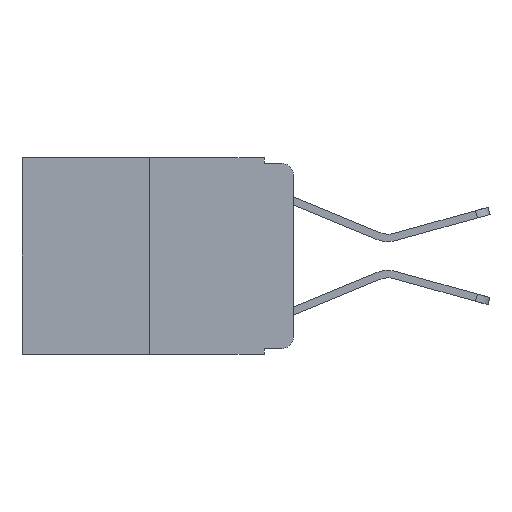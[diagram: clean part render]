
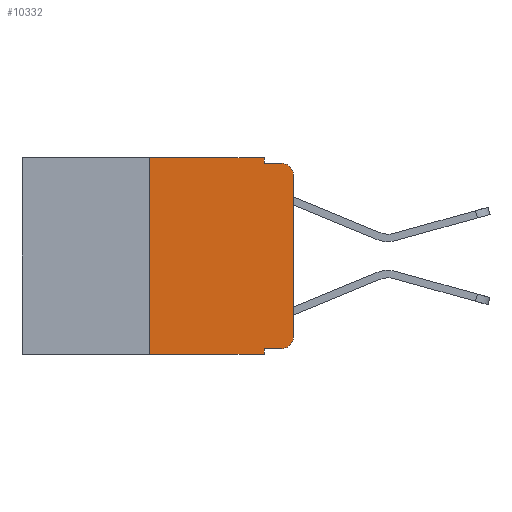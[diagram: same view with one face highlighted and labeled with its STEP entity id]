
A CAD part, left-side view. The second image highlights one B-rep face of the part: STEP entity #10332.
In plain terms, the highlighted planar face has unit normal (-1, 0, 0).
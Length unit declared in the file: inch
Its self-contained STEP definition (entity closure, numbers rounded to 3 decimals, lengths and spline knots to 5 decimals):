
#74 = VECTOR ( 'NONE', #14060, 39.37008 ) ;
#261 = DIRECTION ( 'NONE',  ( 0., -1., 0. ) ) ;
#812 = DIRECTION ( 'NONE',  ( 0., -1., 0. ) ) ;
#1003 = LINE ( 'NONE', #7362, #5046 ) ;
#1047 = VERTEX_POINT ( 'NONE', #14259 ) ;
#1197 = EDGE_LOOP ( 'NONE', ( #1367, #5788, #6211, #12075, #5599, #6016, #3745, #7667, #11487, #1809 ) ) ;
#1241 = DIRECTION ( 'NONE',  ( -1., 0., 0. ) ) ;
#1252 = FACE_OUTER_BOUND ( 'NONE', #1197, .T. ) ;
#1367 = ORIENTED_EDGE ( 'NONE', *, *, #8122, .T. ) ;
#1708 = VERTEX_POINT ( 'NONE', #8657 ) ;
#1809 = ORIENTED_EDGE ( 'NONE', *, *, #1858, .T. ) ;
#1858 = EDGE_CURVE ( 'NONE', #11792, #1047, #4188, .T. ) ;
#2099 = DIRECTION ( 'NONE',  ( 0., 0., 1. ) ) ;
#2276 = CARTESIAN_POINT ( 'NONE',  ( 0., 0.473, -0.343 ) ) ;
#2359 = CARTESIAN_POINT ( 'NONE',  ( 0., 0.25, 0. ) ) ;
#2367 = VECTOR ( 'NONE', #2861, 39.37008 ) ;
#2523 = CARTESIAN_POINT ( 'NONE',  ( 0., 0.02, -0.313 ) ) ;
#2621 = DIRECTION ( 'NONE',  ( 0., 0., -1. ) ) ;
#2690 = VECTOR ( 'NONE', #4657, 39.37008 ) ;
#2783 = EDGE_CURVE ( 'NONE', #15565, #11792, #3538, .T. ) ;
#2861 = DIRECTION ( 'NONE',  ( 0., -1., 0. ) ) ;
#3190 = VERTEX_POINT ( 'NONE', #7915 ) ;
#3263 = LINE ( 'NONE', #11995, #2367 ) ;
#3306 = VERTEX_POINT ( 'NONE', #5562 ) ;
#3320 = CARTESIAN_POINT ( 'NONE',  ( 0., 0.051, 0. ) ) ;
#3538 = LINE ( 'NONE', #13495, #6611 ) ;
#3713 = EDGE_CURVE ( 'NONE', #15565, #3190, #16423, .T. ) ;
#3745 = ORIENTED_EDGE ( 'NONE', *, *, #10357, .T. ) ;
#3856 = VERTEX_POINT ( 'NONE', #9307 ) ;
#3903 = CIRCLE ( 'NONE', #15588, 0.02 ) ;
#4188 = CIRCLE ( 'NONE', #6206, 0.02 ) ;
#4616 = EDGE_CURVE ( 'NONE', #3856, #9664, #1003, .T. ) ;
#4657 = DIRECTION ( 'NONE',  ( 0., 0., -1. ) ) ;
#4954 = CARTESIAN_POINT ( 'NONE',  ( 0., 0.473, 0. ) ) ;
#5046 = VECTOR ( 'NONE', #8669, 39.37008 ) ;
#5477 = EDGE_CURVE ( 'NONE', #15376, #16408, #9713, .T. ) ;
#5562 = CARTESIAN_POINT ( 'NONE',  ( 0., 0.02, -0.01 ) ) ;
#5599 = ORIENTED_EDGE ( 'NONE', *, *, #11134, .F. ) ;
#5788 = ORIENTED_EDGE ( 'NONE', *, *, #7263, .T. ) ;
#5804 = CARTESIAN_POINT ( 'NONE',  ( 0., 0.02, -0.333 ) ) ;
#6016 = ORIENTED_EDGE ( 'NONE', *, *, #4616, .F. ) ;
#6206 = AXIS2_PLACEMENT_3D ( 'NONE', #2523, #1241, #2621 ) ;
#6211 = ORIENTED_EDGE ( 'NONE', *, *, #6350, .F. ) ;
#6261 = DIRECTION ( 'NONE',  ( 1., 0., 0. ) ) ;
#6350 = EDGE_CURVE ( 'NONE', #16408, #3306, #12069, .T. ) ;
#6611 = VECTOR ( 'NONE', #261, 39.37008 ) ;
#7127 = CARTESIAN_POINT ( 'NONE',  ( 0., 0.02, -0.03 ) ) ;
#7263 = EDGE_CURVE ( 'NONE', #1708, #3306, #3903, .T. ) ;
#7362 = CARTESIAN_POINT ( 'NONE',  ( 0., 0.25, 0. ) ) ;
#7667 = ORIENTED_EDGE ( 'NONE', *, *, #3713, .F. ) ;
#7915 = CARTESIAN_POINT ( 'NONE',  ( 0., 0.051, -0.343 ) ) ;
#8122 = EDGE_CURVE ( 'NONE', #1047, #1708, #16113, .T. ) ;
#8379 = CARTESIAN_POINT ( 'NONE',  ( 0., 0.051, -0.333 ) ) ;
#8438 = DIRECTION ( 'NONE',  ( 0., 0., -1. ) ) ;
#8657 = CARTESIAN_POINT ( 'NONE',  ( 0., 0., -0.03 ) ) ;
#8669 = DIRECTION ( 'NONE',  ( 0., 0., 1. ) ) ;
#8786 = PLANE ( 'NONE',  #11282 ) ;
#8804 = CARTESIAN_POINT ( 'NONE',  ( 0., 0.051, -0.01 ) ) ;
#8865 = CARTESIAN_POINT ( 'NONE',  ( 0., 0.051, -0.01 ) ) ;
#8974 = CARTESIAN_POINT ( 'NONE',  ( 0., 0.051, 0. ) ) ;
#9229 = CARTESIAN_POINT ( 'NONE',  ( 0., 0.051, 0. ) ) ;
#9307 = CARTESIAN_POINT ( 'NONE',  ( 0., 0.25, -0.343 ) ) ;
#9664 = VERTEX_POINT ( 'NONE', #2359 ) ;
#9713 = LINE ( 'NONE', #3320, #2690 ) ;
#10143 = VECTOR ( 'NONE', #11548, 39.37008 ) ;
#10332 = ADVANCED_FACE ( 'NONE', ( #1252 ), #8786, .F. ) ;
#10357 = EDGE_CURVE ( 'NONE', #3856, #3190, #10616, .T. ) ;
#10616 = LINE ( 'NONE', #2276, #74 ) ;
#11134 = EDGE_CURVE ( 'NONE', #9664, #15376, #3263, .T. ) ;
#11282 = AXIS2_PLACEMENT_3D ( 'NONE', #4954, #6261, #15233 ) ;
#11487 = ORIENTED_EDGE ( 'NONE', *, *, #2783, .T. ) ;
#11548 = DIRECTION ( 'NONE',  ( 0., 0., -1. ) ) ;
#11792 = VERTEX_POINT ( 'NONE', #5804 ) ;
#11995 = CARTESIAN_POINT ( 'NONE',  ( 0., 0.473, 0. ) ) ;
#12069 = LINE ( 'NONE', #8804, #15416 ) ;
#12075 = ORIENTED_EDGE ( 'NONE', *, *, #5477, .F. ) ;
#12816 = VECTOR ( 'NONE', #2099, 39.37008 ) ;
#13495 = CARTESIAN_POINT ( 'NONE',  ( 0., 0.051, -0.333 ) ) ;
#13794 = CARTESIAN_POINT ( 'NONE',  ( 0., 0., 0. ) ) ;
#14060 = DIRECTION ( 'NONE',  ( 0., -1., 0. ) ) ;
#14259 = CARTESIAN_POINT ( 'NONE',  ( 0., 0., -0.313 ) ) ;
#15233 = DIRECTION ( 'NONE',  ( 0., 0., -1. ) ) ;
#15376 = VERTEX_POINT ( 'NONE', #9229 ) ;
#15416 = VECTOR ( 'NONE', #812, 39.37008 ) ;
#15565 = VERTEX_POINT ( 'NONE', #8379 ) ;
#15588 = AXIS2_PLACEMENT_3D ( 'NONE', #7127, #16010, #8438 ) ;
#16010 = DIRECTION ( 'NONE',  ( -1., 0., 0. ) ) ;
#16113 = LINE ( 'NONE', #13794, #12816 ) ;
#16408 = VERTEX_POINT ( 'NONE', #8865 ) ;
#16423 = LINE ( 'NONE', #8974, #10143 ) ;
